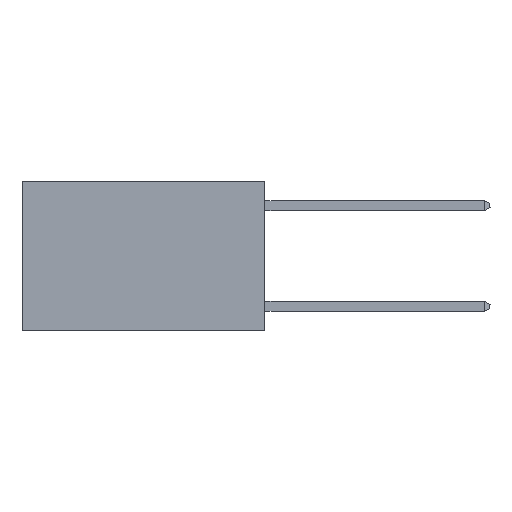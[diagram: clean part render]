
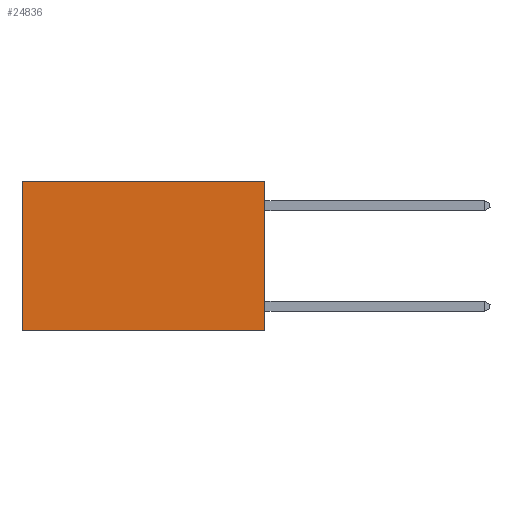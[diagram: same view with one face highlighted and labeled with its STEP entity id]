
A CAD part, left-side view. The second image highlights one B-rep face of the part: STEP entity #24836.
In plain terms, the highlighted planar face has unit normal (-1, 0, 0).
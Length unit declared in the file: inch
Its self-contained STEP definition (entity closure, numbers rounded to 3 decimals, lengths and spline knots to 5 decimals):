
#1092 = LINE ( 'NONE', #3342, #9443 ) ;
#1441 = VECTOR ( 'NONE', #13823, 39.37008 ) ;
#2286 = VECTOR ( 'NONE', #25851, 39.37008 ) ;
#3342 = CARTESIAN_POINT ( 'NONE',  ( 0.2625, 0., 0. ) ) ;
#3648 = PLANE ( 'NONE',  #23023 ) ;
#3791 = DIRECTION ( 'NONE',  ( 1., 0., 0. ) ) ;
#4153 = CARTESIAN_POINT ( 'NONE',  ( 0.2625, 0.6, -0.37 ) ) ;
#4835 = CARTESIAN_POINT ( 'NONE',  ( 0.2625, 0., 0. ) ) ;
#5374 = VERTEX_POINT ( 'NONE', #23271 ) ;
#6769 = LINE ( 'NONE', #7046, #2286 ) ;
#7046 = CARTESIAN_POINT ( 'NONE',  ( 0.2625, 0., 0. ) ) ;
#7270 = EDGE_LOOP ( 'NONE', ( #19934, #19230, #21717, #26294 ) ) ;
#8288 = FACE_OUTER_BOUND ( 'NONE', #7270, .T. ) ;
#8423 = CARTESIAN_POINT ( 'NONE',  ( 0.2625, 0., -0.37 ) ) ;
#8886 = DIRECTION ( 'NONE',  ( 0., 1., 0. ) ) ;
#9443 = VECTOR ( 'NONE', #24262, 39.37008 ) ;
#10384 = CARTESIAN_POINT ( 'NONE',  ( 0.2625, 0., 0. ) ) ;
#11673 = LINE ( 'NONE', #19802, #18754 ) ;
#13008 = EDGE_CURVE ( 'NONE', #15454, #5374, #6769, .T. ) ;
#13823 = DIRECTION ( 'NONE',  ( 0., 0., -1. ) ) ;
#13973 = LINE ( 'NONE', #15937, #1441 ) ;
#15454 = VERTEX_POINT ( 'NONE', #4835 ) ;
#15937 = CARTESIAN_POINT ( 'NONE',  ( 0.2625, 0.6, 0. ) ) ;
#16785 = VERTEX_POINT ( 'NONE', #4153 ) ;
#17429 = EDGE_CURVE ( 'NONE', #24964, #16785, #11673, .T. ) ;
#18754 = VECTOR ( 'NONE', #8886, 39.37008 ) ;
#18921 = DIRECTION ( 'NONE',  ( 0., 0., -1. ) ) ;
#19230 = ORIENTED_EDGE ( 'NONE', *, *, #17429, .F. ) ;
#19802 = CARTESIAN_POINT ( 'NONE',  ( 0.2625, 0., -0.37 ) ) ;
#19934 = ORIENTED_EDGE ( 'NONE', *, *, #23243, .T. ) ;
#21471 = EDGE_CURVE ( 'NONE', #15454, #24964, #1092, .T. ) ;
#21717 = ORIENTED_EDGE ( 'NONE', *, *, #21471, .F. ) ;
#23023 = AXIS2_PLACEMENT_3D ( 'NONE', #10384, #3791, #18921 ) ;
#23243 = EDGE_CURVE ( 'NONE', #5374, #16785, #13973, .T. ) ;
#23271 = CARTESIAN_POINT ( 'NONE',  ( 0.2625, 0.6, 0. ) ) ;
#24262 = DIRECTION ( 'NONE',  ( 0., 0., -1. ) ) ;
#24836 = ADVANCED_FACE ( 'NONE', ( #8288 ), #3648, .F. ) ;
#24964 = VERTEX_POINT ( 'NONE', #8423 ) ;
#25851 = DIRECTION ( 'NONE',  ( 0., 1., 0. ) ) ;
#26294 = ORIENTED_EDGE ( 'NONE', *, *, #13008, .T. ) ;
